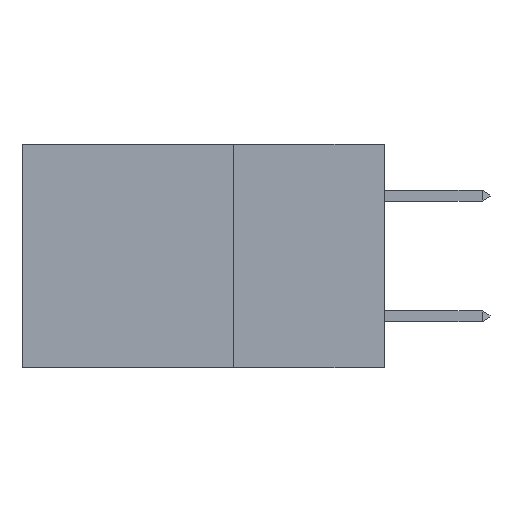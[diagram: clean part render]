
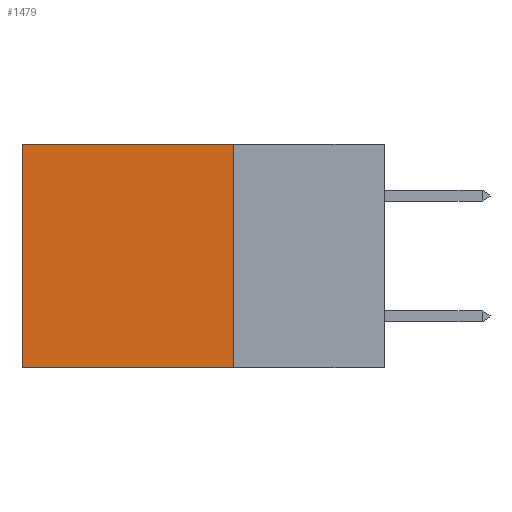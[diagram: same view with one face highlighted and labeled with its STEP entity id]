
A CAD part, left-side view. The second image highlights one B-rep face of the part: STEP entity #1479.
In plain terms, the highlighted planar face has unit normal (-1, 0, 0).
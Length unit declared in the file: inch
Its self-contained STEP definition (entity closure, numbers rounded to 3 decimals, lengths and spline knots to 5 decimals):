
#1374 = CARTESIAN_POINT ( 'NONE',  ( 0.2875, 0.25, 0. ) ) ;
#1479 = ADVANCED_FACE ( 'NONE', ( #7587 ), #4179, .F. ) ;
#2135 = CARTESIAN_POINT ( 'NONE',  ( 0.2875, 0.25, 0. ) ) ;
#2291 = EDGE_LOOP ( 'NONE', ( #14844, #18645, #20608, #5154 ) ) ;
#2491 = EDGE_CURVE ( 'NONE', #13613, #4022, #8084, .T. ) ;
#2879 = DIRECTION ( 'NONE',  ( 0., 1., 0. ) ) ;
#3586 = CARTESIAN_POINT ( 'NONE',  ( 0.2875, 0.25, -0.37 ) ) ;
#4022 = VERTEX_POINT ( 'NONE', #5420 ) ;
#4179 = PLANE ( 'NONE',  #18585 ) ;
#4286 = DIRECTION ( 'NONE',  ( 1., 0., 0. ) ) ;
#4926 = VECTOR ( 'NONE', #16084, 39.37008 ) ;
#5154 = ORIENTED_EDGE ( 'NONE', *, *, #6191, .T. ) ;
#5420 = CARTESIAN_POINT ( 'NONE',  ( 0.2875, 0.6, -0.37 ) ) ;
#5869 = VERTEX_POINT ( 'NONE', #3586 ) ;
#6191 = EDGE_CURVE ( 'NONE', #10983, #13613, #18493, .T. ) ;
#7013 = VECTOR ( 'NONE', #2879, 39.37008 ) ;
#7250 = CARTESIAN_POINT ( 'NONE',  ( 0.2875, 0.6, 0. ) ) ;
#7587 = FACE_OUTER_BOUND ( 'NONE', #2291, .T. ) ;
#8084 = LINE ( 'NONE', #9734, #8786 ) ;
#8786 = VECTOR ( 'NONE', #16500, 39.37008 ) ;
#9508 = LINE ( 'NONE', #16052, #7013 ) ;
#9734 = CARTESIAN_POINT ( 'NONE',  ( 0.2875, 0.6, 0. ) ) ;
#10983 = VERTEX_POINT ( 'NONE', #2135 ) ;
#12578 = CARTESIAN_POINT ( 'NONE',  ( 0.2875, 0.25, 0. ) ) ;
#13613 = VERTEX_POINT ( 'NONE', #7250 ) ;
#14742 = CARTESIAN_POINT ( 'NONE',  ( 0.2875, 0.25, 0. ) ) ;
#14844 = ORIENTED_EDGE ( 'NONE', *, *, #2491, .T. ) ;
#16052 = CARTESIAN_POINT ( 'NONE',  ( 0.2875, 0.25, -0.37 ) ) ;
#16084 = DIRECTION ( 'NONE',  ( 0., 0., -1. ) ) ;
#16143 = VECTOR ( 'NONE', #21484, 39.37008 ) ;
#16500 = DIRECTION ( 'NONE',  ( 0., 0., -1. ) ) ;
#18493 = LINE ( 'NONE', #14742, #16143 ) ;
#18585 = AXIS2_PLACEMENT_3D ( 'NONE', #12578, #4286, #19529 ) ;
#18645 = ORIENTED_EDGE ( 'NONE', *, *, #20021, .F. ) ;
#19529 = DIRECTION ( 'NONE',  ( 0., 0., -1. ) ) ;
#20021 = EDGE_CURVE ( 'NONE', #5869, #4022, #9508, .T. ) ;
#20608 = ORIENTED_EDGE ( 'NONE', *, *, #20966, .F. ) ;
#20966 = EDGE_CURVE ( 'NONE', #10983, #5869, #21375, .T. ) ;
#21375 = LINE ( 'NONE', #1374, #4926 ) ;
#21484 = DIRECTION ( 'NONE',  ( 0., 1., 0. ) ) ;
